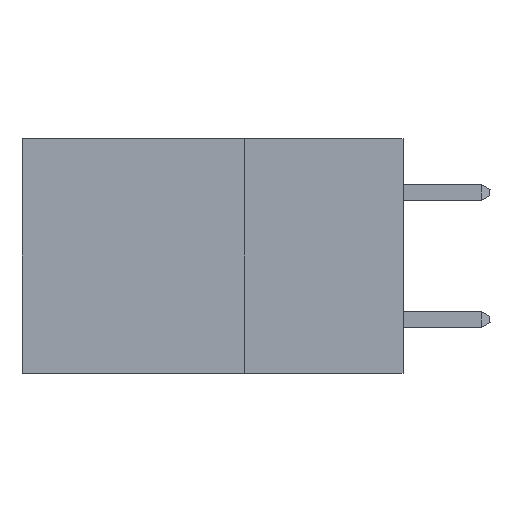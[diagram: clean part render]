
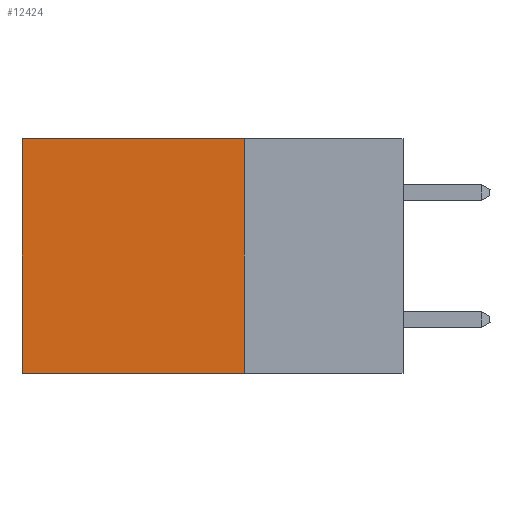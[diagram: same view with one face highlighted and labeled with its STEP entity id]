
A CAD part, left-side view. The second image highlights one B-rep face of the part: STEP entity #12424.
In plain terms, the highlighted planar face has unit normal (-1, 0, 0).
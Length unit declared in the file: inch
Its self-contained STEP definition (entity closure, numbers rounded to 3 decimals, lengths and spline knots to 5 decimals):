
#669 = CARTESIAN_POINT ( 'NONE',  ( 0.2875, 0.25, -0.37 ) ) ;
#745 = LINE ( 'NONE', #12315, #8185 ) ;
#2426 = ORIENTED_EDGE ( 'NONE', *, *, #12396, .T. ) ;
#3361 = VERTEX_POINT ( 'NONE', #9729 ) ;
#4207 = CARTESIAN_POINT ( 'NONE',  ( 0.2875, 0.25, -0.37 ) ) ;
#5733 = VECTOR ( 'NONE', #24811, 39.37008 ) ;
#6961 = CARTESIAN_POINT ( 'NONE',  ( 0.2875, 0.6, 0. ) ) ;
#8185 = VECTOR ( 'NONE', #33173, 39.37008 ) ;
#9729 = CARTESIAN_POINT ( 'NONE',  ( 0.2875, 0.25, 0. ) ) ;
#10694 = LINE ( 'NONE', #11352, #30166 ) ;
#11352 = CARTESIAN_POINT ( 'NONE',  ( 0.2875, 0.25, 0. ) ) ;
#11768 = EDGE_LOOP ( 'NONE', ( #22998, #21452, #23920, #2426 ) ) ;
#12315 = CARTESIAN_POINT ( 'NONE',  ( 0.2875, 0.25, 0. ) ) ;
#12396 = EDGE_CURVE ( 'NONE', #3361, #29648, #10694, .T. ) ;
#12424 = ADVANCED_FACE ( 'NONE', ( #24235 ), #30676, .F. ) ;
#12558 = EDGE_CURVE ( 'NONE', #17442, #25699, #28073, .T. ) ;
#12630 = EDGE_CURVE ( 'NONE', #3361, #17442, #745, .T. ) ;
#13183 = VECTOR ( 'NONE', #22782, 39.37008 ) ;
#14082 = CARTESIAN_POINT ( 'NONE',  ( 0.2875, 0.6, -0.37 ) ) ;
#17442 = VERTEX_POINT ( 'NONE', #669 ) ;
#19575 = EDGE_CURVE ( 'NONE', #29648, #25699, #27669, .T. ) ;
#20814 = CARTESIAN_POINT ( 'NONE',  ( 0.2875, 0.25, 0. ) ) ;
#21452 = ORIENTED_EDGE ( 'NONE', *, *, #12558, .F. ) ;
#22782 = DIRECTION ( 'NONE',  ( 0., 1., 0. ) ) ;
#22998 = ORIENTED_EDGE ( 'NONE', *, *, #19575, .T. ) ;
#23897 = DIRECTION ( 'NONE',  ( 0., 0., -1. ) ) ;
#23920 = ORIENTED_EDGE ( 'NONE', *, *, #12630, .F. ) ;
#24235 = FACE_OUTER_BOUND ( 'NONE', #11768, .T. ) ;
#24811 = DIRECTION ( 'NONE',  ( 0., 0., -1. ) ) ;
#25699 = VERTEX_POINT ( 'NONE', #14082 ) ;
#26372 = DIRECTION ( 'NONE',  ( 1., 0., 0. ) ) ;
#27669 = LINE ( 'NONE', #30844, #5733 ) ;
#28073 = LINE ( 'NONE', #4207, #13183 ) ;
#29648 = VERTEX_POINT ( 'NONE', #6961 ) ;
#29847 = DIRECTION ( 'NONE',  ( 0., 1., 0. ) ) ;
#30166 = VECTOR ( 'NONE', #29847, 39.37008 ) ;
#30305 = AXIS2_PLACEMENT_3D ( 'NONE', #20814, #26372, #23897 ) ;
#30676 = PLANE ( 'NONE',  #30305 ) ;
#30844 = CARTESIAN_POINT ( 'NONE',  ( 0.2875, 0.6, 0. ) ) ;
#33173 = DIRECTION ( 'NONE',  ( 0., 0., -1. ) ) ;
